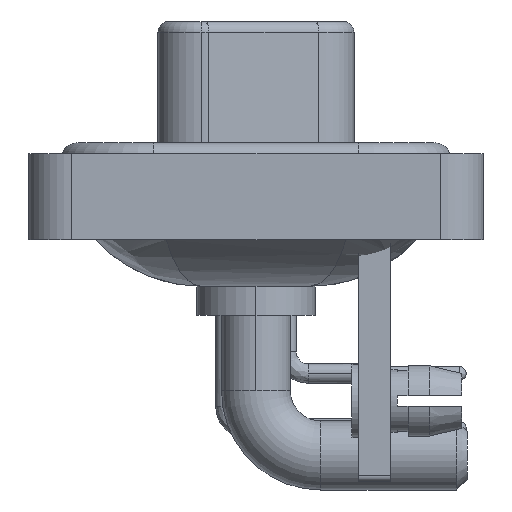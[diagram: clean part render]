
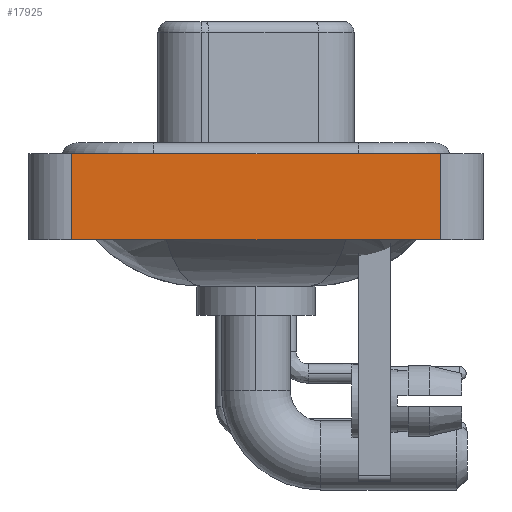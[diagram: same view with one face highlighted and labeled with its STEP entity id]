
A CAD part, left-side view. The second image highlights one B-rep face of the part: STEP entity #17925.
In plain terms, the highlighted planar face has unit normal (-1, 0, 0).
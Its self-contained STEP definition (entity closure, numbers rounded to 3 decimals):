
#277 = DIRECTION ( 'NONE',  ( 0., -1., 0. ) ) ;
#422 = CARTESIAN_POINT ( 'NONE',  ( -7.35, -8.55, 0.4 ) ) ;
#1003 = DIRECTION ( 'NONE',  ( 0., 0., 1. ) ) ;
#1610 = DIRECTION ( 'NONE',  ( 0., 0., 1. ) ) ;
#1819 = LINE ( 'NONE', #16787, #27795 ) ;
#1950 = ORIENTED_EDGE ( 'NONE', *, *, #6867, .T. ) ;
#3346 = ORIENTED_EDGE ( 'NONE', *, *, #4113, .F. ) ;
#4113 = EDGE_CURVE ( 'NONE', #14988, #10032, #19308, .T. ) ;
#6436 = EDGE_LOOP ( 'NONE', ( #1950, #11409, #3346, #19291 ) ) ;
#6867 = EDGE_CURVE ( 'NONE', #25558, #8168, #1819, .T. ) ;
#6873 = LINE ( 'NONE', #422, #10029 ) ;
#6952 = LINE ( 'NONE', #26467, #22321 ) ;
#8168 = VERTEX_POINT ( 'NONE', #14195 ) ;
#10029 = VECTOR ( 'NONE', #277, 1000. ) ;
#10032 = VERTEX_POINT ( 'NONE', #13560 ) ;
#11268 = CARTESIAN_POINT ( 'NONE',  ( -7.35, -8.55, -3.6 ) ) ;
#11409 = ORIENTED_EDGE ( 'NONE', *, *, #22310, .F. ) ;
#13129 = VECTOR ( 'NONE', #1610, 1000. ) ;
#13560 = CARTESIAN_POINT ( 'NONE',  ( -7.35, 8.55, 0.4 ) ) ;
#14078 = PLANE ( 'NONE',  #19951 ) ;
#14195 = CARTESIAN_POINT ( 'NONE',  ( -7.35, -8.55, 0.4 ) ) ;
#14988 = VERTEX_POINT ( 'NONE', #26139 ) ;
#15722 = DIRECTION ( 'NONE',  ( 0., -1., 0. ) ) ;
#16787 = CARTESIAN_POINT ( 'NONE',  ( -7.35, -8.55, -3.6 ) ) ;
#17925 = ADVANCED_FACE ( 'NONE', ( #18561 ), #14078, .T. ) ;
#18561 = FACE_OUTER_BOUND ( 'NONE', #6436, .T. ) ;
#19291 = ORIENTED_EDGE ( 'NONE', *, *, #27231, .T. ) ;
#19308 = LINE ( 'NONE', #26147, #13129 ) ;
#19951 = AXIS2_PLACEMENT_3D ( 'NONE', #22935, #20746, #1003 ) ;
#20746 = DIRECTION ( 'NONE',  ( -1., 0., 0. ) ) ;
#22310 = EDGE_CURVE ( 'NONE', #10032, #8168, #6873, .T. ) ;
#22321 = VECTOR ( 'NONE', #15722, 1000. ) ;
#22935 = CARTESIAN_POINT ( 'NONE',  ( -7.35, -8.55, -3.6 ) ) ;
#25558 = VERTEX_POINT ( 'NONE', #11268 ) ;
#25659 = DIRECTION ( 'NONE',  ( 0., 0., 1. ) ) ;
#26139 = CARTESIAN_POINT ( 'NONE',  ( -7.35, 8.55, -3.6 ) ) ;
#26147 = CARTESIAN_POINT ( 'NONE',  ( -7.35, 8.55, -3.6 ) ) ;
#26467 = CARTESIAN_POINT ( 'NONE',  ( -7.35, -8.55, -3.6 ) ) ;
#27231 = EDGE_CURVE ( 'NONE', #14988, #25558, #6952, .T. ) ;
#27795 = VECTOR ( 'NONE', #25659, 1000. ) ;
